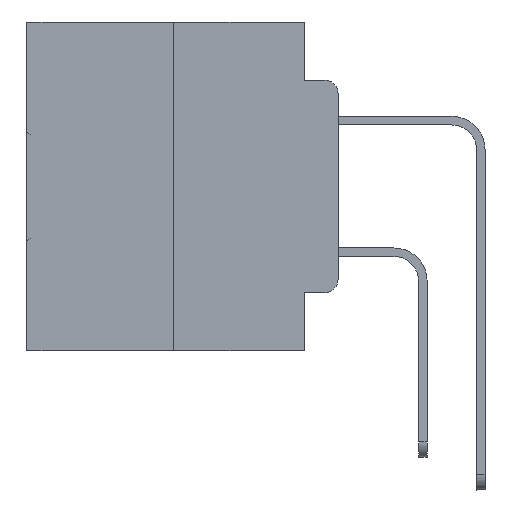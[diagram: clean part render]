
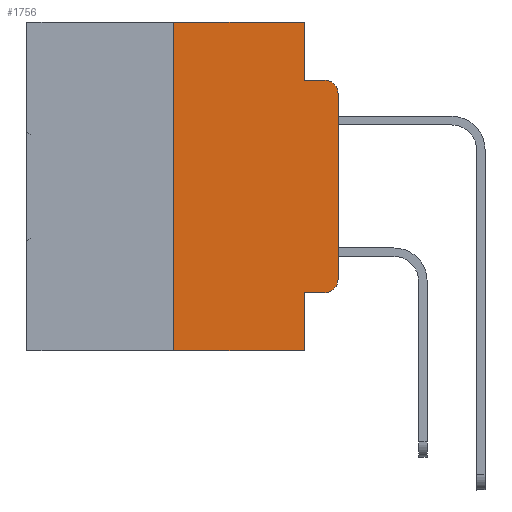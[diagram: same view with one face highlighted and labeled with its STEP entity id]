
A CAD part, left-side view. The second image highlights one B-rep face of the part: STEP entity #1756.
In plain terms, the highlighted planar face has unit normal (-1, 0, 0).
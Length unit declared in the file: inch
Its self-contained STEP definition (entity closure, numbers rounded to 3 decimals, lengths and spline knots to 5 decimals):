
#262 = DIRECTION ( 'NONE',  ( 0., -1., 0. ) ) ;
#1065 = DIRECTION ( 'NONE',  ( 1., 0., 0. ) ) ;
#1756 = ADVANCED_FACE ( 'NONE', ( #22165 ), #14407, .F. ) ;
#2054 = ORIENTED_EDGE ( 'NONE', *, *, #31129, .T. ) ;
#2784 = DIRECTION ( 'NONE',  ( 0., 0., 1. ) ) ;
#3335 = CARTESIAN_POINT ( 'NONE',  ( 0., 0.02, -0.3915 ) ) ;
#3685 = DIRECTION ( 'NONE',  ( 0., 0., -1. ) ) ;
#3688 = CARTESIAN_POINT ( 'NONE',  ( 0., 0., -0.1085 ) ) ;
#4560 = CARTESIAN_POINT ( 'NONE',  ( 0., 0.051, -0.0885 ) ) ;
#4704 = VERTEX_POINT ( 'NONE', #29194 ) ;
#6158 = CARTESIAN_POINT ( 'NONE',  ( 0., 0.051, 0. ) ) ;
#6898 = CARTESIAN_POINT ( 'NONE',  ( 0., 0.051, -0.5 ) ) ;
#7143 = CIRCLE ( 'NONE', #29552, 0.02 ) ;
#7558 = DIRECTION ( 'NONE',  ( 0., 0., -1. ) ) ;
#7731 = ORIENTED_EDGE ( 'NONE', *, *, #34169, .F. ) ;
#7926 = EDGE_CURVE ( 'NONE', #9011, #20832, #21667, .T. ) ;
#7990 = VECTOR ( 'NONE', #262, 39.37008 ) ;
#8248 = VECTOR ( 'NONE', #7558, 39.37008 ) ;
#8441 = DIRECTION ( 'NONE',  ( 0., 0., -1. ) ) ;
#8843 = VECTOR ( 'NONE', #2784, 39.37008 ) ;
#8911 = EDGE_LOOP ( 'NONE', ( #27386, #2054, #22610, #20073, #27805, #7731, #30156, #13337, #10608, #26107 ) ) ;
#9011 = VERTEX_POINT ( 'NONE', #9456 ) ;
#9456 = CARTESIAN_POINT ( 'NONE',  ( 0., 0.25, 0. ) ) ;
#9474 = DIRECTION ( 'NONE',  ( 0., -1., 0. ) ) ;
#9526 = DIRECTION ( 'NONE',  ( 0., 0., -1. ) ) ;
#10608 = ORIENTED_EDGE ( 'NONE', *, *, #21452, .T. ) ;
#10729 = CARTESIAN_POINT ( 'NONE',  ( 0., 0.051, 0. ) ) ;
#11050 = CARTESIAN_POINT ( 'NONE',  ( 0., 0., 0. ) ) ;
#11402 = CARTESIAN_POINT ( 'NONE',  ( 0., 0.02, -0.4115 ) ) ;
#11471 = CARTESIAN_POINT ( 'NONE',  ( 0., 0., -0.3915 ) ) ;
#12266 = LINE ( 'NONE', #22460, #29503 ) ;
#12580 = EDGE_CURVE ( 'NONE', #25670, #30799, #13601, .T. ) ;
#12974 = VECTOR ( 'NONE', #32076, 39.37008 ) ;
#13337 = ORIENTED_EDGE ( 'NONE', *, *, #29187, .F. ) ;
#13601 = LINE ( 'NONE', #24338, #7990 ) ;
#13734 = VERTEX_POINT ( 'NONE', #19172 ) ;
#13908 = VECTOR ( 'NONE', #24089, 39.37008 ) ;
#14407 = PLANE ( 'NONE',  #16635 ) ;
#14506 = VECTOR ( 'NONE', #15281, 39.37008 ) ;
#14893 = CARTESIAN_POINT ( 'NONE',  ( 0., 0.25, -0.5 ) ) ;
#15281 = DIRECTION ( 'NONE',  ( 0., -1., 0. ) ) ;
#15629 = LINE ( 'NONE', #4560, #14506 ) ;
#16635 = AXIS2_PLACEMENT_3D ( 'NONE', #32807, #1065, #9526 ) ;
#16649 = LINE ( 'NONE', #11050, #8843 ) ;
#16821 = CIRCLE ( 'NONE', #24680, 0.02 ) ;
#17042 = DIRECTION ( 'NONE',  ( -1., 0., 0. ) ) ;
#17948 = LINE ( 'NONE', #18296, #13908 ) ;
#18296 = CARTESIAN_POINT ( 'NONE',  ( 0., 0.051, 0. ) ) ;
#18443 = LINE ( 'NONE', #29123, #12974 ) ;
#19172 = CARTESIAN_POINT ( 'NONE',  ( 0., 0.051, -0.0885 ) ) ;
#19629 = VERTEX_POINT ( 'NONE', #3688 ) ;
#20073 = ORIENTED_EDGE ( 'NONE', *, *, #28034, .F. ) ;
#20832 = VERTEX_POINT ( 'NONE', #6158 ) ;
#21263 = VERTEX_POINT ( 'NONE', #11402 ) ;
#21452 = EDGE_CURVE ( 'NONE', #31528, #21263, #12266, .T. ) ;
#21667 = LINE ( 'NONE', #23948, #22904 ) ;
#21890 = CARTESIAN_POINT ( 'NONE',  ( 0., 0.051, -0.4115 ) ) ;
#21976 = CARTESIAN_POINT ( 'NONE',  ( 0., 0.02, -0.1085 ) ) ;
#22019 = DIRECTION ( 'NONE',  ( 0., -1., 0. ) ) ;
#22165 = FACE_OUTER_BOUND ( 'NONE', #8911, .T. ) ;
#22460 = CARTESIAN_POINT ( 'NONE',  ( 0., 0.051, -0.4115 ) ) ;
#22610 = ORIENTED_EDGE ( 'NONE', *, *, #24156, .F. ) ;
#22665 = EDGE_CURVE ( 'NONE', #21263, #30674, #7143, .T. ) ;
#22904 = VECTOR ( 'NONE', #22019, 39.37008 ) ;
#23948 = CARTESIAN_POINT ( 'NONE',  ( 0., 0.473, 0. ) ) ;
#24089 = DIRECTION ( 'NONE',  ( 0., 0., -1. ) ) ;
#24156 = EDGE_CURVE ( 'NONE', #13734, #4704, #15629, .T. ) ;
#24267 = DIRECTION ( 'NONE',  ( -1., 0., 0. ) ) ;
#24305 = EDGE_CURVE ( 'NONE', #30674, #19629, #16649, .T. ) ;
#24338 = CARTESIAN_POINT ( 'NONE',  ( 0., 0.473, -0.5 ) ) ;
#24680 = AXIS2_PLACEMENT_3D ( 'NONE', #21976, #24267, #8441 ) ;
#25670 = VERTEX_POINT ( 'NONE', #14893 ) ;
#26107 = ORIENTED_EDGE ( 'NONE', *, *, #22665, .T. ) ;
#26686 = LINE ( 'NONE', #10729, #8248 ) ;
#27386 = ORIENTED_EDGE ( 'NONE', *, *, #24305, .T. ) ;
#27805 = ORIENTED_EDGE ( 'NONE', *, *, #7926, .F. ) ;
#28034 = EDGE_CURVE ( 'NONE', #20832, #13734, #26686, .T. ) ;
#29123 = CARTESIAN_POINT ( 'NONE',  ( 0., 0.25, 0. ) ) ;
#29187 = EDGE_CURVE ( 'NONE', #31528, #30799, #17948, .T. ) ;
#29194 = CARTESIAN_POINT ( 'NONE',  ( 0., 0.02, -0.0885 ) ) ;
#29503 = VECTOR ( 'NONE', #9474, 39.37008 ) ;
#29552 = AXIS2_PLACEMENT_3D ( 'NONE', #3335, #17042, #3685 ) ;
#30156 = ORIENTED_EDGE ( 'NONE', *, *, #12580, .T. ) ;
#30674 = VERTEX_POINT ( 'NONE', #11471 ) ;
#30799 = VERTEX_POINT ( 'NONE', #6898 ) ;
#31129 = EDGE_CURVE ( 'NONE', #19629, #4704, #16821, .T. ) ;
#31528 = VERTEX_POINT ( 'NONE', #21890 ) ;
#32076 = DIRECTION ( 'NONE',  ( 0., 0., 1. ) ) ;
#32807 = CARTESIAN_POINT ( 'NONE',  ( 0., 0.473, 0. ) ) ;
#34169 = EDGE_CURVE ( 'NONE', #25670, #9011, #18443, .T. ) ;
